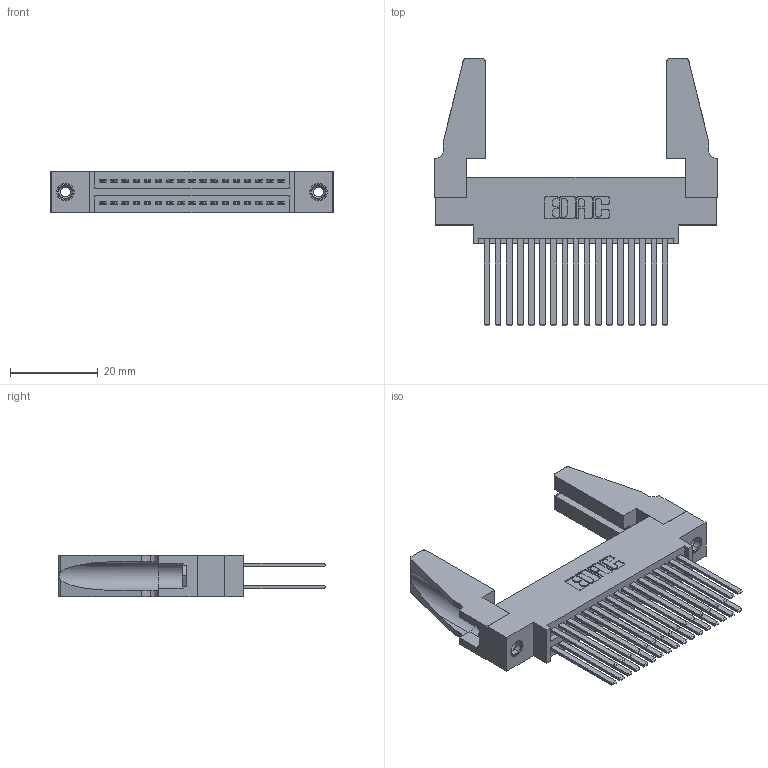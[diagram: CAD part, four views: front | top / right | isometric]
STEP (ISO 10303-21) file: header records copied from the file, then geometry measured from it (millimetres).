
FILE_DESCRIPTION (( 'STEP AP203' ), '1' );
FILE_NAME ('395-034-544-888.STEP', '2019-10-17T18:07:08', ( '' ), ( '' ), 'SwSTEP 2.0', 'SolidWorks 2016', '' );
FILE_SCHEMA (( 'CONFIG_CONTROL_DESIGN' ));
Length unit declared in the file: inch
Products named in the file (5): 345 Part_0.170 Offset - 0.156 Dia-TH; 345-292-001_345-293-144; 345-250-001_345-250-001-102; 345-220-078_345-220-088; 395-034-544-888
Assembly tree (39 placements, depth 2):
  395-034-544-888
    345 Part_0.170 Offset - 0.156 Dia-TH
    345-292-001_345-293-144  x34
    345-250-001_345-250-001-102  x2
    345-220-078_345-220-088  x2
Bounding box: 64.41 x 61.14 x 9.4 mm (x, y, z)
Volume: 9640.9 mm3; surface area: 13621.5 mm2
Topology: 39 solids, 39 shells, 1750 faces, 5121 edges, 3358 vertices
Faces by surface type: plane 1142, cylinder 592, cone 12, torus 4
Entity records: 18800 total; most frequent: CARTESIAN_POINT 3170, ORIENTED_EDGE 3064, DIRECTION 2828, EDGE_CURVE 1532, LINE 1294, VECTOR 1294, VERTEX_POINT 1014, AXIS2_PLACEMENT_3D 767
